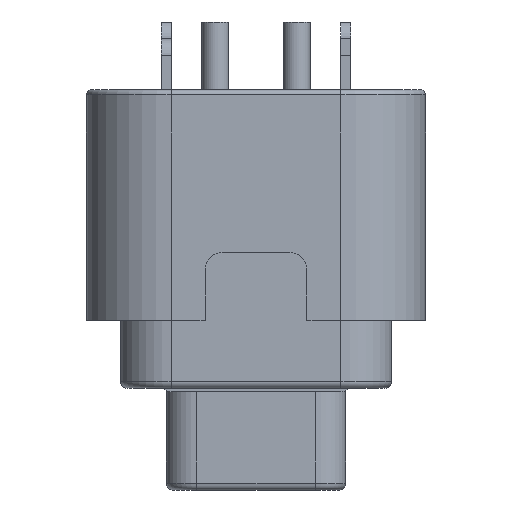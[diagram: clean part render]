
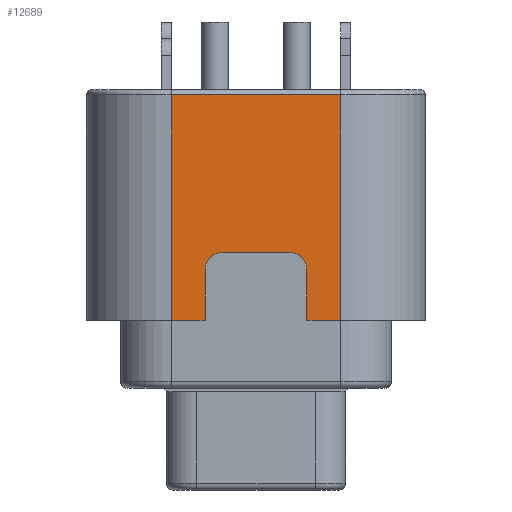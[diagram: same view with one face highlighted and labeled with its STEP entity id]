
A CAD part, left-side view. The second image highlights one B-rep face of the part: STEP entity #12689.
In plain terms, the highlighted planar face has unit normal (-1, 0, 0).
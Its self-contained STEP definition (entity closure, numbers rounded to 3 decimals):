
#7 = LINE ( 'NONE', #11083, #15254 ) ;
#148 = LINE ( 'NONE', #11226, #34140 ) ;
#888 = CARTESIAN_POINT ( 'NONE',  ( -19.7, -1.5, 2.2 ) ) ;
#1537 = FACE_OUTER_BOUND ( 'NONE', #25488, .T. ) ;
#1795 = VERTEX_POINT ( 'NONE', #32605 ) ;
#2300 = EDGE_CURVE ( 'NONE', #8858, #26569, #148, .T. ) ;
#3081 = DIRECTION ( 'NONE',  ( 0., 0., 1. ) ) ;
#3221 = EDGE_CURVE ( 'NONE', #19763, #3948, #25986, .T. ) ;
#3620 = VERTEX_POINT ( 'NONE', #888 ) ;
#3948 = VERTEX_POINT ( 'NONE', #9421 ) ;
#4151 = LINE ( 'NONE', #15193, #29107 ) ;
#4579 = DIRECTION ( 'NONE',  ( 0., 0., 1. ) ) ;
#5036 = VERTEX_POINT ( 'NONE', #22229 ) ;
#5765 = ORIENTED_EDGE ( 'NONE', *, *, #16405, .T. ) ;
#6137 = DIRECTION ( 'NONE',  ( 0., -1., 0. ) ) ;
#6579 = DIRECTION ( 'NONE',  ( 0., 1., 0. ) ) ;
#7128 = AXIS2_PLACEMENT_3D ( 'NONE', #23601, #34642, #9899 ) ;
#8108 = EDGE_CURVE ( 'NONE', #24651, #8858, #10684, .T. ) ;
#8278 = VECTOR ( 'NONE', #3081, 1000. ) ;
#8858 = VERTEX_POINT ( 'NONE', #29016 ) ;
#9421 = CARTESIAN_POINT ( 'NONE',  ( -19.7, 1., 4.2 ) ) ;
#9489 = VECTOR ( 'NONE', #6137, 1000. ) ;
#9801 = EDGE_CURVE ( 'NONE', #3620, #33603, #35431, .T. ) ;
#9850 = CARTESIAN_POINT ( 'NONE',  ( -19.7, -2.5, 2.2 ) ) ;
#9899 = DIRECTION ( 'NONE',  ( 0., 1., 0. ) ) ;
#10409 = AXIS2_PLACEMENT_3D ( 'NONE', #20304, #31330, #6579 ) ;
#10684 = LINE ( 'NONE', #21683, #10980 ) ;
#10690 = CARTESIAN_POINT ( 'NONE',  ( -19.7, -1.5, 2.2 ) ) ;
#10980 = VECTOR ( 'NONE', #32710, 1000. ) ;
#11083 = CARTESIAN_POINT ( 'NONE',  ( -19.7, -1.5, 3.7 ) ) ;
#11226 = CARTESIAN_POINT ( 'NONE',  ( -19.7, 2.5, 8.85 ) ) ;
#12195 = EDGE_CURVE ( 'NONE', #24330, #3620, #7, .T. ) ;
#12599 = PLANE ( 'NONE',  #7128 ) ;
#12689 = ADVANCED_FACE ( 'NONE', ( #1537 ), #12599, .F. ) ;
#12885 = CARTESIAN_POINT ( 'NONE',  ( -19.7, 1.5, 3.7 ) ) ;
#13120 = EDGE_CURVE ( 'NONE', #1795, #24330, #14666, .T. ) ;
#14086 = CARTESIAN_POINT ( 'NONE',  ( -19.7, -2.5, 2.2 ) ) ;
#14493 = ORIENTED_EDGE ( 'NONE', *, *, #16860, .T. ) ;
#14666 = CIRCLE ( 'NONE', #34844, 0.5 ) ;
#15133 = EDGE_CURVE ( 'NONE', #1795, #3948, #4151, .T. ) ;
#15193 = CARTESIAN_POINT ( 'NONE',  ( -19.7, -1., 4.2 ) ) ;
#15254 = VECTOR ( 'NONE', #22085, 1000. ) ;
#16198 = CARTESIAN_POINT ( 'NONE',  ( -19.7, 2.5, 2.2 ) ) ;
#16405 = EDGE_CURVE ( 'NONE', #5036, #19763, #16847, .T. ) ;
#16847 = LINE ( 'NONE', #27845, #8278 ) ;
#16860 = EDGE_CURVE ( 'NONE', #26569, #5036, #19866, .T. ) ;
#17805 = VECTOR ( 'NONE', #21690, 1000. ) ;
#17905 = EDGE_CURVE ( 'NONE', #33603, #24651, #34593, .T. ) ;
#18324 = CARTESIAN_POINT ( 'NONE',  ( -19.7, -1., 3.7 ) ) ;
#19763 = VERTEX_POINT ( 'NONE', #12885 ) ;
#19866 = LINE ( 'NONE', #30895, #9489 ) ;
#20198 = ORIENTED_EDGE ( 'NONE', *, *, #17905, .T. ) ;
#20304 = CARTESIAN_POINT ( 'NONE',  ( -19.7, 1., 3.7 ) ) ;
#20857 = DIRECTION ( 'NONE',  ( 0., 0., 1. ) ) ;
#21286 = ORIENTED_EDGE ( 'NONE', *, *, #8108, .T. ) ;
#21683 = CARTESIAN_POINT ( 'NONE',  ( -19.7, -2.5, 8.85 ) ) ;
#21690 = DIRECTION ( 'NONE',  ( 0., -1., 0. ) ) ;
#22085 = DIRECTION ( 'NONE',  ( 0., 0., -1. ) ) ;
#22213 = VECTOR ( 'NONE', #20857, 1000. ) ;
#22225 = DIRECTION ( 'NONE',  ( 0., 0., -1. ) ) ;
#22229 = CARTESIAN_POINT ( 'NONE',  ( -19.7, 1.5, 2.2 ) ) ;
#23601 = CARTESIAN_POINT ( 'NONE',  ( -19.7, 0., 5.525 ) ) ;
#24330 = VERTEX_POINT ( 'NONE', #25196 ) ;
#24651 = VERTEX_POINT ( 'NONE', #33443 ) ;
#24868 = ORIENTED_EDGE ( 'NONE', *, *, #3221, .T. ) ;
#25196 = CARTESIAN_POINT ( 'NONE',  ( -19.7, -1.5, 3.7 ) ) ;
#25488 = EDGE_LOOP ( 'NONE', ( #34671, #20198, #21286, #29008, #14493, #5765, #24868, #28881, #29092, #34656 ) ) ;
#25986 = CIRCLE ( 'NONE', #10409, 0.5 ) ;
#26203 = DIRECTION ( 'NONE',  ( 0., 1., 0. ) ) ;
#26569 = VERTEX_POINT ( 'NONE', #16198 ) ;
#27845 = CARTESIAN_POINT ( 'NONE',  ( -19.7, 1.5, 2.2 ) ) ;
#28881 = ORIENTED_EDGE ( 'NONE', *, *, #15133, .F. ) ;
#29008 = ORIENTED_EDGE ( 'NONE', *, *, #2300, .T. ) ;
#29016 = CARTESIAN_POINT ( 'NONE',  ( -19.7, 2.5, 8.85 ) ) ;
#29092 = ORIENTED_EDGE ( 'NONE', *, *, #13120, .T. ) ;
#29107 = VECTOR ( 'NONE', #26203, 1000. ) ;
#29329 = DIRECTION ( 'NONE',  ( 1., 0., 0. ) ) ;
#30895 = CARTESIAN_POINT ( 'NONE',  ( -19.7, 2.5, 2.2 ) ) ;
#31330 = DIRECTION ( 'NONE',  ( 1., 0., 0. ) ) ;
#32605 = CARTESIAN_POINT ( 'NONE',  ( -19.7, -1., 4.2 ) ) ;
#32710 = DIRECTION ( 'NONE',  ( 0., 1., 0. ) ) ;
#33443 = CARTESIAN_POINT ( 'NONE',  ( -19.7, -2.5, 8.85 ) ) ;
#33603 = VERTEX_POINT ( 'NONE', #14086 ) ;
#34140 = VECTOR ( 'NONE', #22225, 1000. ) ;
#34593 = LINE ( 'NONE', #9850, #22213 ) ;
#34642 = DIRECTION ( 'NONE',  ( 1., 0., 0. ) ) ;
#34656 = ORIENTED_EDGE ( 'NONE', *, *, #12195, .T. ) ;
#34671 = ORIENTED_EDGE ( 'NONE', *, *, #9801, .T. ) ;
#34844 = AXIS2_PLACEMENT_3D ( 'NONE', #18324, #29329, #4579 ) ;
#35431 = LINE ( 'NONE', #10690, #17805 ) ;
